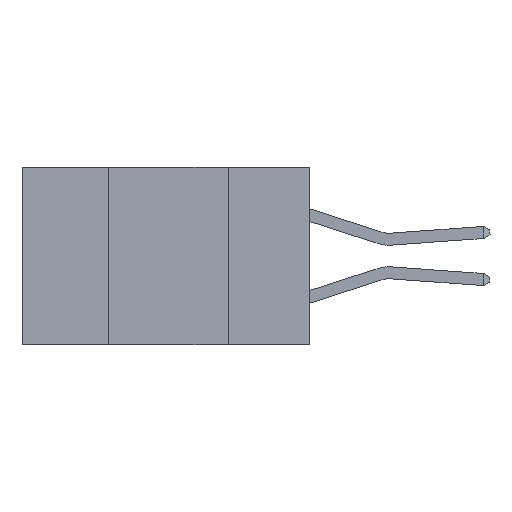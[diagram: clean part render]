
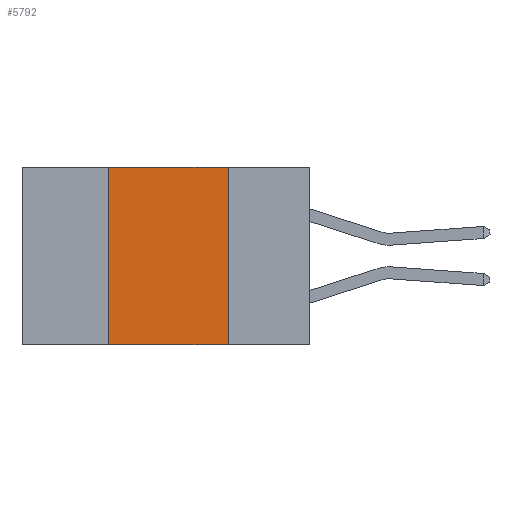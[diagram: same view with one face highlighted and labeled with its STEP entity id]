
A CAD part, left-side view. The second image highlights one B-rep face of the part: STEP entity #5792.
In plain terms, the highlighted planar face has unit normal (-1, 0, 0).
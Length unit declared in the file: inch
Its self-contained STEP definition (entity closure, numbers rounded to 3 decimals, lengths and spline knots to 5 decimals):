
#330 = CARTESIAN_POINT ( 'NONE',  ( 0., 0.42, -0.37 ) ) ;
#465 = ORIENTED_EDGE ( 'NONE', *, *, #9648, .T. ) ;
#469 = LINE ( 'NONE', #12401, #4150 ) ;
#2146 = LINE ( 'NONE', #12652, #5408 ) ;
#2503 = ORIENTED_EDGE ( 'NONE', *, *, #5578, .F. ) ;
#3858 = EDGE_CURVE ( 'NONE', #7767, #9481, #5868, .T. ) ;
#4150 = VECTOR ( 'NONE', #4393, 39.37008 ) ;
#4393 = DIRECTION ( 'NONE',  ( 0., -1., 0. ) ) ;
#4649 = CARTESIAN_POINT ( 'NONE',  ( 0., 0.17, 0. ) ) ;
#5408 = VECTOR ( 'NONE', #9990, 39.37008 ) ;
#5510 = ORIENTED_EDGE ( 'NONE', *, *, #10480, .F. ) ;
#5578 = EDGE_CURVE ( 'NONE', #15905, #11115, #11231, .T. ) ;
#5792 = ADVANCED_FACE ( 'NONE', ( #8321 ), #9269, .F. ) ;
#5868 = LINE ( 'NONE', #13276, #16267 ) ;
#6687 = CARTESIAN_POINT ( 'NONE',  ( 0., 0.42, 0. ) ) ;
#7407 = ORIENTED_EDGE ( 'NONE', *, *, #3858, .F. ) ;
#7733 = VECTOR ( 'NONE', #10941, 39.37008 ) ;
#7767 = VERTEX_POINT ( 'NONE', #330 ) ;
#8321 = FACE_OUTER_BOUND ( 'NONE', #9847, .T. ) ;
#8572 = CARTESIAN_POINT ( 'NONE',  ( 0., 0.17, -0.37 ) ) ;
#9150 = DIRECTION ( 'NONE',  ( 0., 0., -1. ) ) ;
#9167 = DIRECTION ( 'NONE',  ( 1., 0., 0. ) ) ;
#9246 = CARTESIAN_POINT ( 'NONE',  ( 0., 0.6, 0. ) ) ;
#9269 = PLANE ( 'NONE',  #15222 ) ;
#9481 = VERTEX_POINT ( 'NONE', #6687 ) ;
#9648 = EDGE_CURVE ( 'NONE', #7767, #11115, #469, .T. ) ;
#9847 = EDGE_LOOP ( 'NONE', ( #2503, #5510, #7407, #465 ) ) ;
#9990 = DIRECTION ( 'NONE',  ( 0., -1., 0. ) ) ;
#10480 = EDGE_CURVE ( 'NONE', #9481, #15905, #2146, .T. ) ;
#10941 = DIRECTION ( 'NONE',  ( 0., 0., -1. ) ) ;
#10977 = CARTESIAN_POINT ( 'NONE',  ( 0., 0.17, 0. ) ) ;
#11115 = VERTEX_POINT ( 'NONE', #8572 ) ;
#11231 = LINE ( 'NONE', #10977, #7733 ) ;
#12401 = CARTESIAN_POINT ( 'NONE',  ( 0., 0.6, -0.37 ) ) ;
#12652 = CARTESIAN_POINT ( 'NONE',  ( 0., 0.6, 0. ) ) ;
#12742 = DIRECTION ( 'NONE',  ( 0., 0., 1. ) ) ;
#13276 = CARTESIAN_POINT ( 'NONE',  ( 0., 0.42, 0. ) ) ;
#15222 = AXIS2_PLACEMENT_3D ( 'NONE', #9246, #9167, #9150 ) ;
#15905 = VERTEX_POINT ( 'NONE', #4649 ) ;
#16267 = VECTOR ( 'NONE', #12742, 39.37008 ) ;
